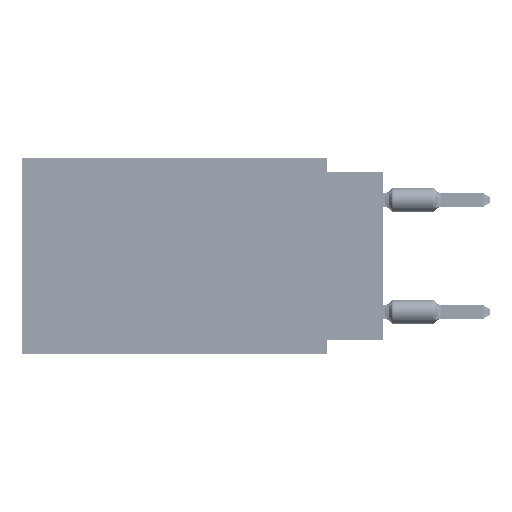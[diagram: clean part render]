
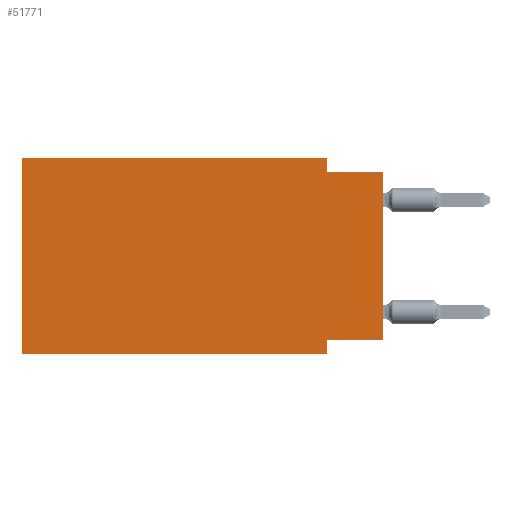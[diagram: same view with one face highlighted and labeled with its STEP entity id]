
A CAD part, left-side view. The second image highlights one B-rep face of the part: STEP entity #51771.
In plain terms, the highlighted planar face has unit normal (-1, 0, 0).
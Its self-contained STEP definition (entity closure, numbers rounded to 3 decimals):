
#1871 = CARTESIAN_POINT ( 'NONE',  ( 0., 16.383, 0. ) ) ;
#2418 = ORIENTED_EDGE ( 'NONE', *, *, #43943, .F. ) ;
#3217 = EDGE_CURVE ( 'NONE', #76746, #32283, #63278, .T. ) ;
#5269 = VERTEX_POINT ( 'NONE', #18432 ) ;
#7231 = DIRECTION ( 'NONE',  ( 0., 0., -1. ) ) ;
#9328 = DIRECTION ( 'NONE',  ( 0., 1., 0. ) ) ;
#9897 = AXIS2_PLACEMENT_3D ( 'NONE', #11936, #60705, #24127 ) ;
#10581 = VERTEX_POINT ( 'NONE', #63183 ) ;
#11936 = CARTESIAN_POINT ( 'NONE',  ( 0., 16.383, 0. ) ) ;
#13164 = ORIENTED_EDGE ( 'NONE', *, *, #37689, .F. ) ;
#13674 = DIRECTION ( 'NONE',  ( 0., -1., 0. ) ) ;
#13820 = DIRECTION ( 'NONE',  ( 0., -1., 0. ) ) ;
#15371 = VECTOR ( 'NONE', #7231, 1000. ) ;
#18432 = CARTESIAN_POINT ( 'NONE',  ( 0., 2.54, 0. ) ) ;
#23565 = CARTESIAN_POINT ( 'NONE',  ( 0., 2.54, -8.89 ) ) ;
#24127 = DIRECTION ( 'NONE',  ( 0., 0., -1. ) ) ;
#24959 = CARTESIAN_POINT ( 'NONE',  ( 0., 16.383, 0. ) ) ;
#26324 = VECTOR ( 'NONE', #9328, 1000. ) ;
#26525 = LINE ( 'NONE', #40737, #46896 ) ;
#27202 = CARTESIAN_POINT ( 'NONE',  ( 0., 0., -8.255 ) ) ;
#29093 = ORIENTED_EDGE ( 'NONE', *, *, #52286, .F. ) ;
#29244 = VERTEX_POINT ( 'NONE', #44874 ) ;
#32283 = VERTEX_POINT ( 'NONE', #37333 ) ;
#33543 = DIRECTION ( 'NONE',  ( 0., 0., 1. ) ) ;
#34959 = EDGE_LOOP ( 'NONE', ( #61543, #29093, #76497, #2418, #35052, #41771, #13164, #68440 ) ) ;
#35038 = CARTESIAN_POINT ( 'NONE',  ( 0., 16.383, -8.89 ) ) ;
#35052 = ORIENTED_EDGE ( 'NONE', *, *, #79886, .F. ) ;
#36320 = FACE_OUTER_BOUND ( 'NONE', #34959, .T. ) ;
#37333 = CARTESIAN_POINT ( 'NONE',  ( 0., 0., -0.635 ) ) ;
#37689 = EDGE_CURVE ( 'NONE', #10581, #48968, #26525, .T. ) ;
#39000 = LINE ( 'NONE', #27202, #26324 ) ;
#40737 = CARTESIAN_POINT ( 'NONE',  ( 0., 2.54, -8.89 ) ) ;
#41551 = VECTOR ( 'NONE', #57173, 1000. ) ;
#41771 = ORIENTED_EDGE ( 'NONE', *, *, #79777, .T. ) ;
#42021 = PLANE ( 'NONE',  #9897 ) ;
#42728 = LINE ( 'NONE', #50813, #44983 ) ;
#43735 = DIRECTION ( 'NONE',  ( 0., -1., 0. ) ) ;
#43943 = EDGE_CURVE ( 'NONE', #68930, #5269, #62451, .T. ) ;
#44874 = CARTESIAN_POINT ( 'NONE',  ( 0., 2.54, -0.635 ) ) ;
#44928 = LINE ( 'NONE', #1871, #72504 ) ;
#44983 = VECTOR ( 'NONE', #13820, 1000. ) ;
#46896 = VECTOR ( 'NONE', #51717, 1000. ) ;
#48968 = VERTEX_POINT ( 'NONE', #23565 ) ;
#50813 = CARTESIAN_POINT ( 'NONE',  ( 0., 0., -0.635 ) ) ;
#51488 = CARTESIAN_POINT ( 'NONE',  ( 0., 0., 0. ) ) ;
#51717 = DIRECTION ( 'NONE',  ( 0., 0., -1. ) ) ;
#51771 = ADVANCED_FACE ( 'NONE', ( #36320 ), #42021, .F. ) ;
#52286 = EDGE_CURVE ( 'NONE', #29244, #32283, #42728, .T. ) ;
#53340 = VERTEX_POINT ( 'NONE', #35038 ) ;
#57173 = DIRECTION ( 'NONE',  ( 0., 0., 1. ) ) ;
#60699 = VECTOR ( 'NONE', #13674, 1000. ) ;
#60705 = DIRECTION ( 'NONE',  ( 1., 0., 0. ) ) ;
#61236 = LINE ( 'NONE', #74626, #62110 ) ;
#61543 = ORIENTED_EDGE ( 'NONE', *, *, #3217, .T. ) ;
#62110 = VECTOR ( 'NONE', #43735, 1000. ) ;
#62451 = LINE ( 'NONE', #63256, #60699 ) ;
#63183 = CARTESIAN_POINT ( 'NONE',  ( 0., 2.54, -8.255 ) ) ;
#63256 = CARTESIAN_POINT ( 'NONE',  ( 0., 16.383, 0. ) ) ;
#63278 = LINE ( 'NONE', #51488, #41551 ) ;
#66177 = EDGE_CURVE ( 'NONE', #76746, #10581, #39000, .T. ) ;
#68440 = ORIENTED_EDGE ( 'NONE', *, *, #66177, .F. ) ;
#68930 = VERTEX_POINT ( 'NONE', #24959 ) ;
#69803 = CARTESIAN_POINT ( 'NONE',  ( 0., 2.54, 0. ) ) ;
#72504 = VECTOR ( 'NONE', #33543, 1000. ) ;
#74626 = CARTESIAN_POINT ( 'NONE',  ( 0., 16.383, -8.89 ) ) ;
#74898 = CARTESIAN_POINT ( 'NONE',  ( 0., 0., -8.255 ) ) ;
#76497 = ORIENTED_EDGE ( 'NONE', *, *, #79447, .F. ) ;
#76746 = VERTEX_POINT ( 'NONE', #74898 ) ;
#77116 = LINE ( 'NONE', #69803, #15371 ) ;
#79447 = EDGE_CURVE ( 'NONE', #5269, #29244, #77116, .T. ) ;
#79777 = EDGE_CURVE ( 'NONE', #53340, #48968, #61236, .T. ) ;
#79886 = EDGE_CURVE ( 'NONE', #53340, #68930, #44928, .T. ) ;
